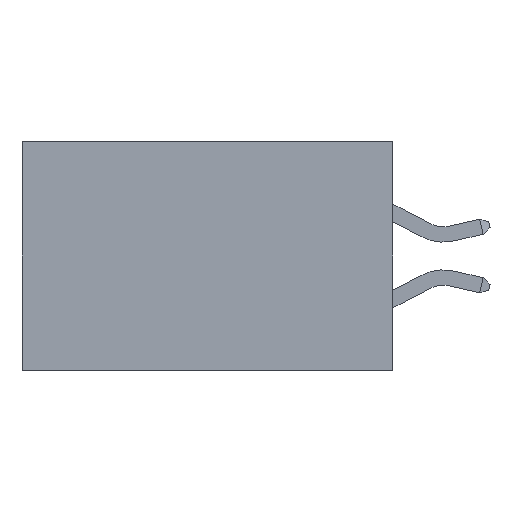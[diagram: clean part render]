
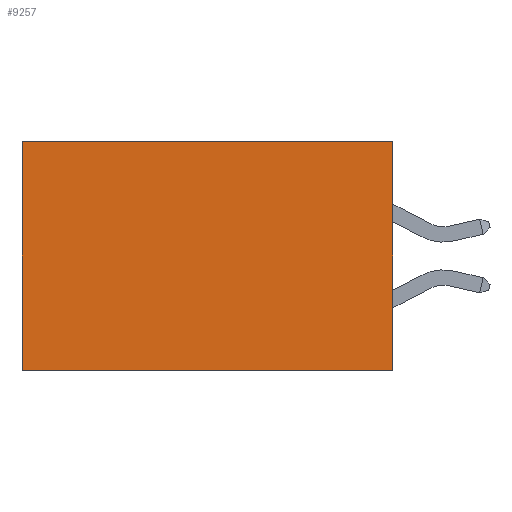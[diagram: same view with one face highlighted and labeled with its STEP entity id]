
A CAD part, left-side view. The second image highlights one B-rep face of the part: STEP entity #9257.
In plain terms, the highlighted planar face has unit normal (-1, 0, 0).
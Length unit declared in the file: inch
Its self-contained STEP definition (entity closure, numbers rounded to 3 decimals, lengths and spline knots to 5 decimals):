
#186 = DIRECTION ( 'NONE',  ( 0., 1., 0. ) ) ;
#192 = ORIENTED_EDGE ( 'NONE', *, *, #10060, .T. ) ;
#319 = LINE ( 'NONE', #8985, #6380 ) ;
#326 = CARTESIAN_POINT ( 'NONE',  ( 0.2875, 0.6, -0.37 ) ) ;
#836 = ORIENTED_EDGE ( 'NONE', *, *, #4582, .T. ) ;
#1033 = FACE_OUTER_BOUND ( 'NONE', #9098, .T. ) ;
#1221 = CARTESIAN_POINT ( 'NONE',  ( 0.2875, 0.6, 0. ) ) ;
#1640 = ORIENTED_EDGE ( 'NONE', *, *, #2047, .F. ) ;
#1738 = VERTEX_POINT ( 'NONE', #4947 ) ;
#1825 = ORIENTED_EDGE ( 'NONE', *, *, #2071, .F. ) ;
#2047 = EDGE_CURVE ( 'NONE', #1738, #8285, #2629, .T. ) ;
#2071 = EDGE_CURVE ( 'NONE', #3718, #1738, #319, .T. ) ;
#2197 = AXIS2_PLACEMENT_3D ( 'NONE', #9418, #4089, #10327 ) ;
#2325 = PLANE ( 'NONE',  #2197 ) ;
#2629 = LINE ( 'NONE', #7296, #9990 ) ;
#2843 = LINE ( 'NONE', #1221, #2982 ) ;
#2982 = VECTOR ( 'NONE', #8422, 39.37008 ) ;
#3408 = DIRECTION ( 'NONE',  ( 0., 1., 0. ) ) ;
#3718 = VERTEX_POINT ( 'NONE', #4191 ) ;
#4089 = DIRECTION ( 'NONE',  ( 1., 0., 0. ) ) ;
#4191 = CARTESIAN_POINT ( 'NONE',  ( 0.2875, 0., 0. ) ) ;
#4582 = EDGE_CURVE ( 'NONE', #5433, #8285, #2843, .T. ) ;
#4854 = VECTOR ( 'NONE', #3408, 39.37008 ) ;
#4947 = CARTESIAN_POINT ( 'NONE',  ( 0.2875, 0., -0.37 ) ) ;
#5433 = VERTEX_POINT ( 'NONE', #6170 ) ;
#6071 = CARTESIAN_POINT ( 'NONE',  ( 0.2875, 0., 0. ) ) ;
#6170 = CARTESIAN_POINT ( 'NONE',  ( 0.2875, 0.6, 0. ) ) ;
#6380 = VECTOR ( 'NONE', #9192, 39.37008 ) ;
#7296 = CARTESIAN_POINT ( 'NONE',  ( 0.2875, 0., -0.37 ) ) ;
#8285 = VERTEX_POINT ( 'NONE', #326 ) ;
#8422 = DIRECTION ( 'NONE',  ( 0., 0., -1. ) ) ;
#8985 = CARTESIAN_POINT ( 'NONE',  ( 0.2875, 0., 0. ) ) ;
#9098 = EDGE_LOOP ( 'NONE', ( #836, #1640, #1825, #192 ) ) ;
#9192 = DIRECTION ( 'NONE',  ( 0., 0., -1. ) ) ;
#9257 = ADVANCED_FACE ( 'NONE', ( #1033 ), #2325, .F. ) ;
#9418 = CARTESIAN_POINT ( 'NONE',  ( 0.2875, 0., 0. ) ) ;
#9872 = LINE ( 'NONE', #6071, #4854 ) ;
#9990 = VECTOR ( 'NONE', #186, 39.37008 ) ;
#10060 = EDGE_CURVE ( 'NONE', #3718, #5433, #9872, .T. ) ;
#10327 = DIRECTION ( 'NONE',  ( 0., 0., -1. ) ) ;
